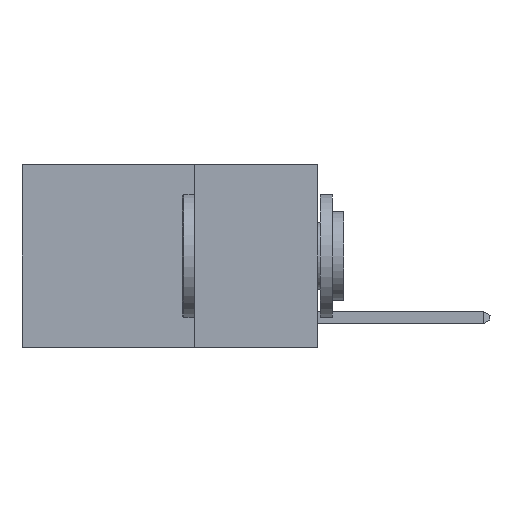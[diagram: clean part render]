
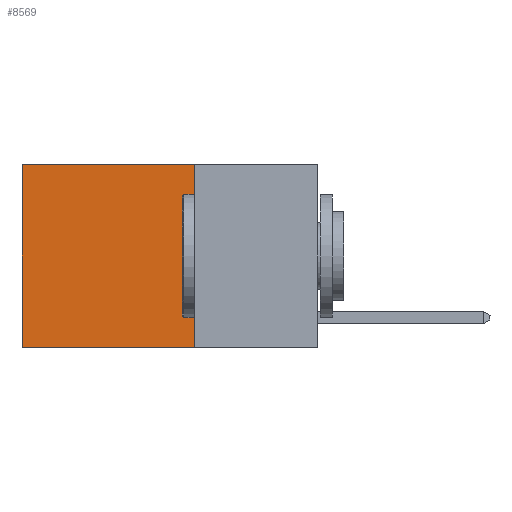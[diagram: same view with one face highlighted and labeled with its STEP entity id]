
A CAD part, left-side view. The second image highlights one B-rep face of the part: STEP entity #8569.
In plain terms, the highlighted planar face has unit normal (-1, 0, 0).
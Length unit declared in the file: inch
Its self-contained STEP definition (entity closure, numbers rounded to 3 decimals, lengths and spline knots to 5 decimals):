
#226 = PLANE ( 'NONE',  #12354 ) ;
#738 = LINE ( 'NONE', #17679, #16577 ) ;
#931 = CARTESIAN_POINT ( 'NONE',  ( 0.2625, 0.25, 0. ) ) ;
#974 = ORIENTED_EDGE ( 'NONE', *, *, #7126, .T. ) ;
#1285 = DIRECTION ( 'NONE',  ( 0., 1., 0. ) ) ;
#1659 = CARTESIAN_POINT ( 'NONE',  ( 0.2625, 0.6, 0. ) ) ;
#2123 = VECTOR ( 'NONE', #16923, 39.37008 ) ;
#2293 = VERTEX_POINT ( 'NONE', #931 ) ;
#2481 = LINE ( 'NONE', #4275, #17687 ) ;
#4275 = CARTESIAN_POINT ( 'NONE',  ( 0.2625, 0.6, 0. ) ) ;
#4332 = VERTEX_POINT ( 'NONE', #1659 ) ;
#4978 = DIRECTION ( 'NONE',  ( 0., 1., 0. ) ) ;
#5900 = VERTEX_POINT ( 'NONE', #9313 ) ;
#6874 = CARTESIAN_POINT ( 'NONE',  ( 0.2625, 0.25, 0. ) ) ;
#7126 = EDGE_CURVE ( 'NONE', #2293, #4332, #15064, .T. ) ;
#7277 = EDGE_CURVE ( 'NONE', #4332, #16037, #2481, .T. ) ;
#8233 = EDGE_LOOP ( 'NONE', ( #12197, #16537, #11136, #974 ) ) ;
#8320 = CARTESIAN_POINT ( 'NONE',  ( 0.2625, 0.25, 0. ) ) ;
#8425 = LINE ( 'NONE', #6874, #2123 ) ;
#8449 = DIRECTION ( 'NONE',  ( 0., 0., -1. ) ) ;
#8513 = DIRECTION ( 'NONE',  ( 1., 0., 0. ) ) ;
#8569 = ADVANCED_FACE ( 'NONE', ( #9218 ), #226, .F. ) ;
#9218 = FACE_OUTER_BOUND ( 'NONE', #8233, .T. ) ;
#9313 = CARTESIAN_POINT ( 'NONE',  ( 0.2625, 0.25, -0.37 ) ) ;
#9613 = CARTESIAN_POINT ( 'NONE',  ( 0.2625, 0.25, 0. ) ) ;
#11136 = ORIENTED_EDGE ( 'NONE', *, *, #17390, .F. ) ;
#11408 = VECTOR ( 'NONE', #1285, 39.37008 ) ;
#11603 = CARTESIAN_POINT ( 'NONE',  ( 0.2625, 0.6, -0.37 ) ) ;
#12038 = EDGE_CURVE ( 'NONE', #5900, #16037, #738, .T. ) ;
#12197 = ORIENTED_EDGE ( 'NONE', *, *, #7277, .T. ) ;
#12354 = AXIS2_PLACEMENT_3D ( 'NONE', #8320, #8513, #8449 ) ;
#12705 = DIRECTION ( 'NONE',  ( 0., 0., -1. ) ) ;
#15064 = LINE ( 'NONE', #9613, #11408 ) ;
#16037 = VERTEX_POINT ( 'NONE', #11603 ) ;
#16537 = ORIENTED_EDGE ( 'NONE', *, *, #12038, .F. ) ;
#16577 = VECTOR ( 'NONE', #4978, 39.37008 ) ;
#16923 = DIRECTION ( 'NONE',  ( 0., 0., -1. ) ) ;
#17390 = EDGE_CURVE ( 'NONE', #2293, #5900, #8425, .T. ) ;
#17679 = CARTESIAN_POINT ( 'NONE',  ( 0.2625, 0.25, -0.37 ) ) ;
#17687 = VECTOR ( 'NONE', #12705, 39.37008 ) ;
